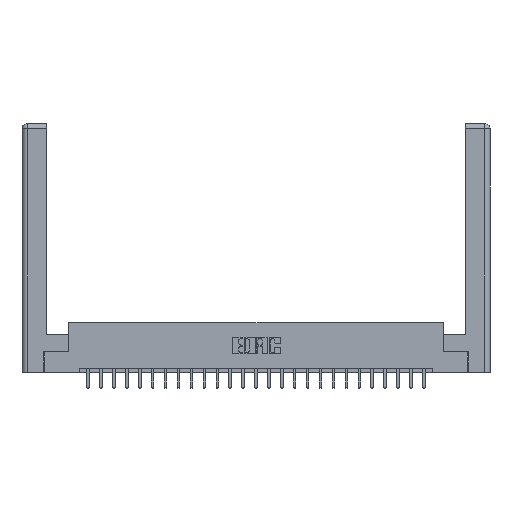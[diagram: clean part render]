
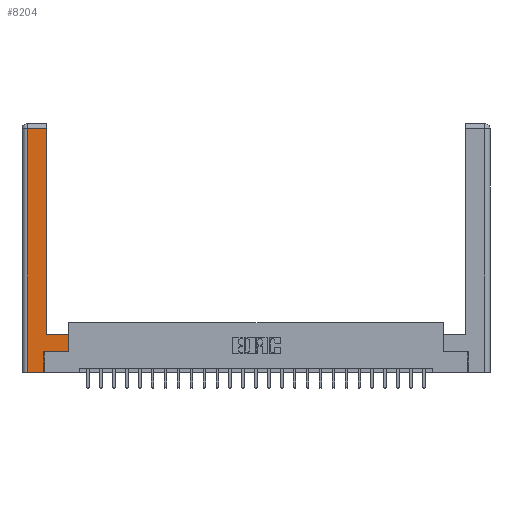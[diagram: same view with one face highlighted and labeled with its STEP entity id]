
A CAD part, top view. The second image highlights one B-rep face of the part: STEP entity #8204.
In plain terms, the highlighted planar face has unit normal (0, 0, 1).
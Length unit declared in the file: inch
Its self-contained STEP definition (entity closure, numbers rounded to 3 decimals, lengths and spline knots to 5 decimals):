
#993 = VECTOR ( 'NONE', #1286, 39.37008 ) ;
#1165 = DIRECTION ( 'NONE',  ( -1., 0., 0. ) ) ;
#1286 = DIRECTION ( 'NONE',  ( -1., 0., 0. ) ) ;
#1642 = CARTESIAN_POINT ( 'NONE',  ( 0.265, 0., 0. ) ) ;
#1983 = EDGE_CURVE ( 'NONE', #22065, #16227, #8677, .T. ) ;
#2303 = CARTESIAN_POINT ( 'NONE',  ( 0.265, 0., 0. ) ) ;
#2456 = ORIENTED_EDGE ( 'NONE', *, *, #1983, .T. ) ;
#2672 = CARTESIAN_POINT ( 'NONE',  ( 0.295, 0.45, 0. ) ) ;
#2737 = LINE ( 'NONE', #8891, #13590 ) ;
#3090 = CARTESIAN_POINT ( 'NONE',  ( 0.295, 2.94, 0. ) ) ;
#3843 = DIRECTION ( 'NONE',  ( 0., 1., 0. ) ) ;
#4105 = ORIENTED_EDGE ( 'NONE', *, *, #21654, .T. ) ;
#4235 = FACE_OUTER_BOUND ( 'NONE', #10150, .T. ) ;
#4600 = DIRECTION ( 'NONE',  ( -1., 0., 0. ) ) ;
#4901 = VERTEX_POINT ( 'NONE', #3090 ) ;
#6265 = ORIENTED_EDGE ( 'NONE', *, *, #21719, .T. ) ;
#6296 = VECTOR ( 'NONE', #13806, 39.37008 ) ;
#7159 = CARTESIAN_POINT ( 'NONE',  ( 0., 0., 0. ) ) ;
#7180 = CARTESIAN_POINT ( 'NONE',  ( 0.265, 0.245, 0. ) ) ;
#7416 = EDGE_CURVE ( 'NONE', #23475, #16686, #2737, .T. ) ;
#8204 = ADVANCED_FACE ( 'NONE', ( #4235 ), #20994, .F. ) ;
#8451 = CARTESIAN_POINT ( 'NONE',  ( 0.295, 3., 0. ) ) ;
#8677 = LINE ( 'NONE', #2303, #23931 ) ;
#8891 = CARTESIAN_POINT ( 'NONE',  ( 0.565, 0.45, 0. ) ) ;
#9169 = CARTESIAN_POINT ( 'NONE',  ( 0.0615, 2.94, 0. ) ) ;
#9499 = LINE ( 'NONE', #12212, #17912 ) ;
#9808 = LINE ( 'NONE', #8451, #17268 ) ;
#9834 = CARTESIAN_POINT ( 'NONE',  ( 0.565, 0.45, 0. ) ) ;
#10150 = EDGE_LOOP ( 'NONE', ( #18324, #19132, #14549, #2456, #14360, #6265, #21455, #4105 ) ) ;
#10324 = VERTEX_POINT ( 'NONE', #16099 ) ;
#10942 = CARTESIAN_POINT ( 'NONE',  ( 0.295, 0.45, 0. ) ) ;
#11369 = AXIS2_PLACEMENT_3D ( 'NONE', #7159, #15283, #1165 ) ;
#11861 = CARTESIAN_POINT ( 'NONE',  ( 0.0615, 0., 0. ) ) ;
#12212 = CARTESIAN_POINT ( 'NONE',  ( 0.265, 0.245, 0. ) ) ;
#12383 = DIRECTION ( 'NONE',  ( 0., 1., 0. ) ) ;
#12558 = LINE ( 'NONE', #10942, #17216 ) ;
#13590 = VECTOR ( 'NONE', #3843, 39.37008 ) ;
#13683 = CARTESIAN_POINT ( 'NONE',  ( 0.0615, 0., 0. ) ) ;
#13806 = DIRECTION ( 'NONE',  ( 1., 0., 0. ) ) ;
#14312 = LINE ( 'NONE', #9169, #993 ) ;
#14360 = ORIENTED_EDGE ( 'NONE', *, *, #20115, .T. ) ;
#14549 = ORIENTED_EDGE ( 'NONE', *, *, #22173, .T. ) ;
#15283 = DIRECTION ( 'NONE',  ( 0., 0., -1. ) ) ;
#16099 = CARTESIAN_POINT ( 'NONE',  ( 0.0615, 2.94, 0. ) ) ;
#16227 = VERTEX_POINT ( 'NONE', #1642 ) ;
#16328 = DIRECTION ( 'NONE',  ( 1., 0., 0. ) ) ;
#16686 = VERTEX_POINT ( 'NONE', #9834 ) ;
#16908 = LINE ( 'NONE', #19207, #6296 ) ;
#17216 = VECTOR ( 'NONE', #4600, 39.37008 ) ;
#17268 = VECTOR ( 'NONE', #18312, 39.37008 ) ;
#17912 = VECTOR ( 'NONE', #12383, 39.37008 ) ;
#18124 = VERTEX_POINT ( 'NONE', #7180 ) ;
#18137 = EDGE_CURVE ( 'NONE', #4901, #10324, #14312, .T. ) ;
#18238 = VERTEX_POINT ( 'NONE', #2672 ) ;
#18312 = DIRECTION ( 'NONE',  ( 0., 1., 0. ) ) ;
#18324 = ORIENTED_EDGE ( 'NONE', *, *, #24234, .T. ) ;
#19132 = ORIENTED_EDGE ( 'NONE', *, *, #18137, .T. ) ;
#19207 = CARTESIAN_POINT ( 'NONE',  ( 0.565, 0.245, 0. ) ) ;
#19627 = LINE ( 'NONE', #13683, #21762 ) ;
#20115 = EDGE_CURVE ( 'NONE', #16227, #18124, #9499, .T. ) ;
#20994 = PLANE ( 'NONE',  #11369 ) ;
#21455 = ORIENTED_EDGE ( 'NONE', *, *, #7416, .T. ) ;
#21654 = EDGE_CURVE ( 'NONE', #16686, #18238, #12558, .T. ) ;
#21719 = EDGE_CURVE ( 'NONE', #18124, #23475, #16908, .T. ) ;
#21762 = VECTOR ( 'NONE', #23736, 39.37008 ) ;
#22065 = VERTEX_POINT ( 'NONE', #11861 ) ;
#22169 = CARTESIAN_POINT ( 'NONE',  ( 0.565, 0.245, 0. ) ) ;
#22173 = EDGE_CURVE ( 'NONE', #10324, #22065, #19627, .T. ) ;
#23475 = VERTEX_POINT ( 'NONE', #22169 ) ;
#23736 = DIRECTION ( 'NONE',  ( 0., -1., 0. ) ) ;
#23931 = VECTOR ( 'NONE', #16328, 39.37008 ) ;
#24234 = EDGE_CURVE ( 'NONE', #18238, #4901, #9808, .T. ) ;
